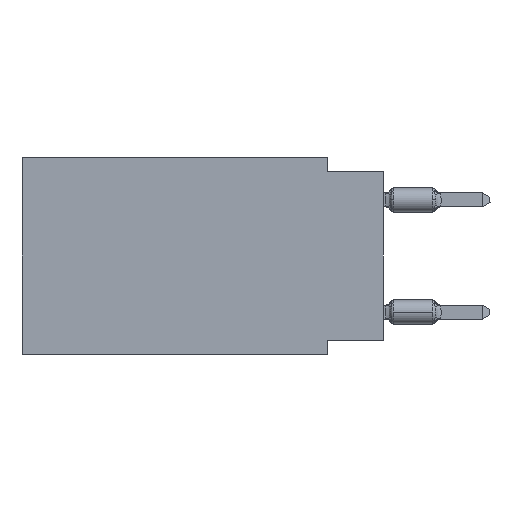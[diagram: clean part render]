
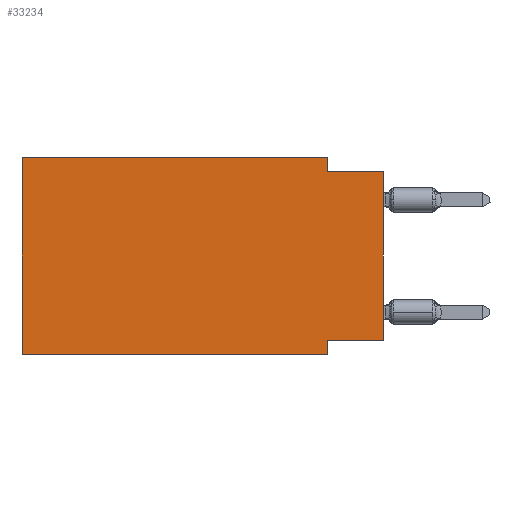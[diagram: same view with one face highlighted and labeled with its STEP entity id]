
A CAD part, left-side view. The second image highlights one B-rep face of the part: STEP entity #33234.
In plain terms, the highlighted planar face has unit normal (-1, 0, 0).
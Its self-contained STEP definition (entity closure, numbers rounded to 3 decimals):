
#42 = CARTESIAN_POINT ( 'NONE',  ( 0., 0., -8.255 ) ) ;
#1228 = EDGE_LOOP ( 'NONE', ( #21008, #16459, #32190, #35789, #18834, #26708, #20668, #14961 ) ) ;
#1305 = EDGE_CURVE ( 'NONE', #12645, #17444, #23792, .T. ) ;
#1697 = VECTOR ( 'NONE', #13235, 1000. ) ;
#2116 = LINE ( 'NONE', #21264, #1697 ) ;
#2766 = CARTESIAN_POINT ( 'NONE',  ( 0., 16.383, -8.89 ) ) ;
#4526 = CARTESIAN_POINT ( 'NONE',  ( 0., 16.383, 0. ) ) ;
#6029 = CARTESIAN_POINT ( 'NONE',  ( 0., 16.383, 0. ) ) ;
#6050 = LINE ( 'NONE', #22830, #34138 ) ;
#6061 = EDGE_CURVE ( 'NONE', #9500, #6639, #30508, .T. ) ;
#6076 = CARTESIAN_POINT ( 'NONE',  ( 0., 2.54, 0. ) ) ;
#6126 = VECTOR ( 'NONE', #29442, 1000. ) ;
#6639 = VERTEX_POINT ( 'NONE', #22424 ) ;
#8021 = CARTESIAN_POINT ( 'NONE',  ( 0., 2.54, -8.89 ) ) ;
#8403 = LINE ( 'NONE', #6029, #13963 ) ;
#8827 = DIRECTION ( 'NONE',  ( 0., 0., -1. ) ) ;
#9200 = VECTOR ( 'NONE', #27419, 1000. ) ;
#9500 = VERTEX_POINT ( 'NONE', #21790 ) ;
#9683 = CARTESIAN_POINT ( 'NONE',  ( 0., 2.54, 0. ) ) ;
#11291 = EDGE_CURVE ( 'NONE', #9500, #29227, #2116, .T. ) ;
#11896 = LINE ( 'NONE', #6076, #34215 ) ;
#11982 = EDGE_CURVE ( 'NONE', #23226, #12645, #8403, .T. ) ;
#12642 = DIRECTION ( 'NONE',  ( 0., 0., -1. ) ) ;
#12645 = VERTEX_POINT ( 'NONE', #4526 ) ;
#12666 = CARTESIAN_POINT ( 'NONE',  ( 0., 0., -0.635 ) ) ;
#13235 = DIRECTION ( 'NONE',  ( 0., 0., 1. ) ) ;
#13892 = DIRECTION ( 'NONE',  ( 0., -1., 0. ) ) ;
#13963 = VECTOR ( 'NONE', #22806, 1000. ) ;
#14340 = VERTEX_POINT ( 'NONE', #20140 ) ;
#14961 = ORIENTED_EDGE ( 'NONE', *, *, #6061, .F. ) ;
#15766 = VERTEX_POINT ( 'NONE', #8021 ) ;
#16459 = ORIENTED_EDGE ( 'NONE', *, *, #19104, .F. ) ;
#17444 = VERTEX_POINT ( 'NONE', #9683 ) ;
#17660 = CARTESIAN_POINT ( 'NONE',  ( 0., 0., -0.635 ) ) ;
#17769 = PLANE ( 'NONE',  #21516 ) ;
#18314 = CARTESIAN_POINT ( 'NONE',  ( 0., 16.383, 0. ) ) ;
#18834 = ORIENTED_EDGE ( 'NONE', *, *, #11982, .F. ) ;
#19104 = EDGE_CURVE ( 'NONE', #14340, #29227, #20376, .T. ) ;
#19309 = VECTOR ( 'NONE', #28951, 1000. ) ;
#19826 = VECTOR ( 'NONE', #13892, 1000. ) ;
#20140 = CARTESIAN_POINT ( 'NONE',  ( 0., 2.54, -0.635 ) ) ;
#20376 = LINE ( 'NONE', #17660, #19309 ) ;
#20668 = ORIENTED_EDGE ( 'NONE', *, *, #23218, .F. ) ;
#21008 = ORIENTED_EDGE ( 'NONE', *, *, #11291, .T. ) ;
#21264 = CARTESIAN_POINT ( 'NONE',  ( 0., 0., 0. ) ) ;
#21516 = AXIS2_PLACEMENT_3D ( 'NONE', #18314, #29262, #12642 ) ;
#21790 = CARTESIAN_POINT ( 'NONE',  ( 0., 0., -8.255 ) ) ;
#22424 = CARTESIAN_POINT ( 'NONE',  ( 0., 2.54, -8.255 ) ) ;
#22806 = DIRECTION ( 'NONE',  ( 0., 0., 1. ) ) ;
#22830 = CARTESIAN_POINT ( 'NONE',  ( 0., 2.54, -8.89 ) ) ;
#23218 = EDGE_CURVE ( 'NONE', #6639, #15766, #6050, .T. ) ;
#23226 = VERTEX_POINT ( 'NONE', #28671 ) ;
#23428 = CARTESIAN_POINT ( 'NONE',  ( 0., 16.383, 0. ) ) ;
#23792 = LINE ( 'NONE', #23428, #6126 ) ;
#25124 = EDGE_CURVE ( 'NONE', #17444, #14340, #11896, .T. ) ;
#26708 = ORIENTED_EDGE ( 'NONE', *, *, #34741, .T. ) ;
#27419 = DIRECTION ( 'NONE',  ( 0., 1., 0. ) ) ;
#27752 = LINE ( 'NONE', #2766, #19826 ) ;
#28671 = CARTESIAN_POINT ( 'NONE',  ( 0., 16.383, -8.89 ) ) ;
#28951 = DIRECTION ( 'NONE',  ( 0., -1., 0. ) ) ;
#29227 = VERTEX_POINT ( 'NONE', #12666 ) ;
#29262 = DIRECTION ( 'NONE',  ( 1., 0., 0. ) ) ;
#29442 = DIRECTION ( 'NONE',  ( 0., -1., 0. ) ) ;
#30508 = LINE ( 'NONE', #42, #9200 ) ;
#31209 = DIRECTION ( 'NONE',  ( 0., 0., -1. ) ) ;
#32190 = ORIENTED_EDGE ( 'NONE', *, *, #25124, .F. ) ;
#33234 = ADVANCED_FACE ( 'NONE', ( #34358 ), #17769, .F. ) ;
#34138 = VECTOR ( 'NONE', #31209, 1000. ) ;
#34215 = VECTOR ( 'NONE', #8827, 1000. ) ;
#34358 = FACE_OUTER_BOUND ( 'NONE', #1228, .T. ) ;
#34741 = EDGE_CURVE ( 'NONE', #23226, #15766, #27752, .T. ) ;
#35789 = ORIENTED_EDGE ( 'NONE', *, *, #1305, .F. ) ;
